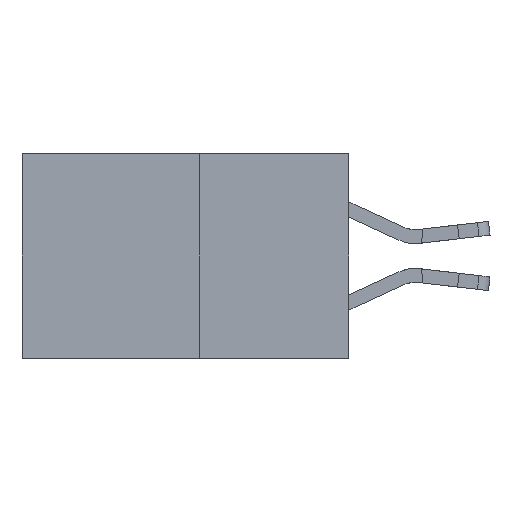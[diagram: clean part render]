
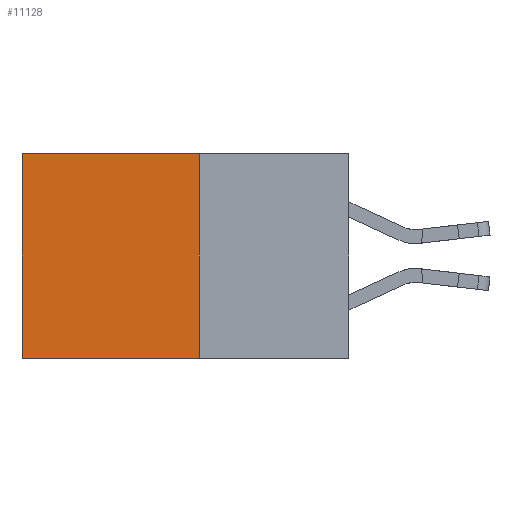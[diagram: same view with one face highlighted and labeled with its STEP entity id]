
A CAD part, left-side view. The second image highlights one B-rep face of the part: STEP entity #11128.
In plain terms, the highlighted planar face has unit normal (-1, 0, 0).
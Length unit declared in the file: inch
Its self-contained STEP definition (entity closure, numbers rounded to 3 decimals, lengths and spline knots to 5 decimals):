
#477 = ORIENTED_EDGE ( 'NONE', *, *, #17121, .F. ) ;
#1071 = CARTESIAN_POINT ( 'NONE',  ( 0.277, 0.27, -0.37 ) ) ;
#1285 = DIRECTION ( 'NONE',  ( 0., 0., -1. ) ) ;
#2106 = CARTESIAN_POINT ( 'NONE',  ( 0.277, 0.59, 0. ) ) ;
#2159 = DIRECTION ( 'NONE',  ( 1., 0., 0. ) ) ;
#3603 = AXIS2_PLACEMENT_3D ( 'NONE', #10407, #2159, #11798 ) ;
#3978 = ORIENTED_EDGE ( 'NONE', *, *, #11357, .F. ) ;
#4359 = VERTEX_POINT ( 'NONE', #1071 ) ;
#4794 = CARTESIAN_POINT ( 'NONE',  ( 0.277, 0.27, -0.37 ) ) ;
#4806 = DIRECTION ( 'NONE',  ( 0., 1., 0. ) ) ;
#4922 = CARTESIAN_POINT ( 'NONE',  ( 0.277, 0.27, 0. ) ) ;
#5468 = EDGE_CURVE ( 'NONE', #10555, #14849, #16970, .T. ) ;
#5697 = EDGE_CURVE ( 'NONE', #7230, #10555, #6315, .T. ) ;
#5870 = VECTOR ( 'NONE', #4806, 39.37008 ) ;
#6175 = DIRECTION ( 'NONE',  ( 0., 1., 0. ) ) ;
#6315 = LINE ( 'NONE', #4922, #5870 ) ;
#6575 = VECTOR ( 'NONE', #1285, 39.37008 ) ;
#6791 = VECTOR ( 'NONE', #6175, 39.37008 ) ;
#7020 = FACE_OUTER_BOUND ( 'NONE', #12470, .T. ) ;
#7230 = VERTEX_POINT ( 'NONE', #9627 ) ;
#7821 = ORIENTED_EDGE ( 'NONE', *, *, #5697, .T. ) ;
#9340 = ORIENTED_EDGE ( 'NONE', *, *, #5468, .T. ) ;
#9627 = CARTESIAN_POINT ( 'NONE',  ( 0.277, 0.27, 0. ) ) ;
#9767 = VECTOR ( 'NONE', #10759, 39.37008 ) ;
#10245 = CARTESIAN_POINT ( 'NONE',  ( 0.277, 0.59, -0.37 ) ) ;
#10407 = CARTESIAN_POINT ( 'NONE',  ( 0.277, 0.27, -0.37 ) ) ;
#10555 = VERTEX_POINT ( 'NONE', #2106 ) ;
#10759 = DIRECTION ( 'NONE',  ( 0., 0., -1. ) ) ;
#10802 = CARTESIAN_POINT ( 'NONE',  ( 0.277, 0.59, -0.37 ) ) ;
#11128 = ADVANCED_FACE ( 'NONE', ( #7020 ), #17163, .F. ) ;
#11357 = EDGE_CURVE ( 'NONE', #4359, #14849, #17605, .T. ) ;
#11798 = DIRECTION ( 'NONE',  ( 0., 0., -1. ) ) ;
#12470 = EDGE_LOOP ( 'NONE', ( #9340, #3978, #477, #7821 ) ) ;
#14849 = VERTEX_POINT ( 'NONE', #10245 ) ;
#16970 = LINE ( 'NONE', #10802, #9767 ) ;
#17000 = LINE ( 'NONE', #17609, #6575 ) ;
#17121 = EDGE_CURVE ( 'NONE', #7230, #4359, #17000, .T. ) ;
#17163 = PLANE ( 'NONE',  #3603 ) ;
#17605 = LINE ( 'NONE', #4794, #6791 ) ;
#17609 = CARTESIAN_POINT ( 'NONE',  ( 0.277, 0.27, -0.37 ) ) ;
